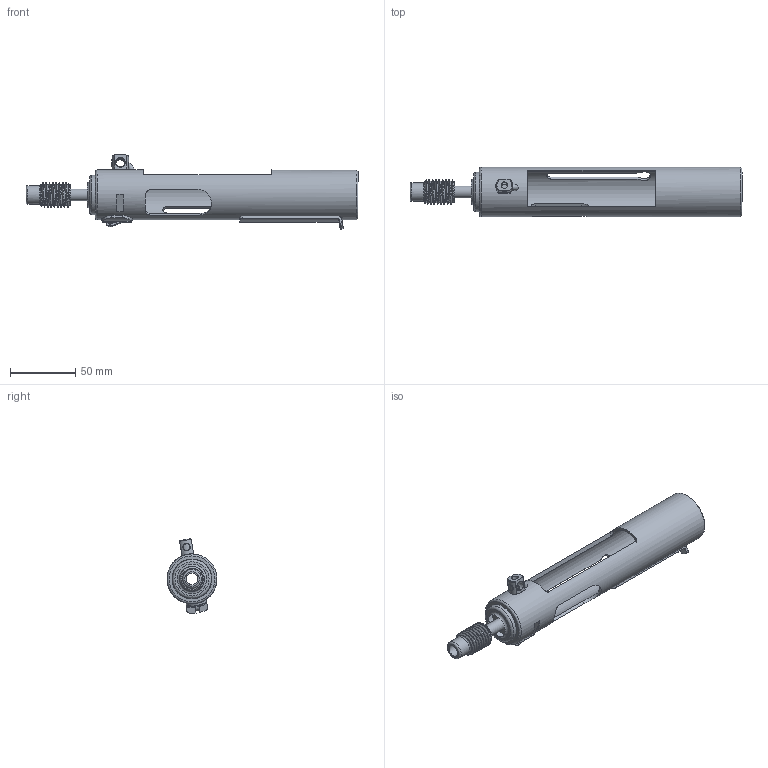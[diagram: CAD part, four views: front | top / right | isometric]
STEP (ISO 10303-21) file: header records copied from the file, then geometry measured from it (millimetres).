
FILE_DESCRIPTION(/* description */ (''),/* implementation_level */ '2;1');
FILE_NAME(/* name */ 'TwoStripedMini.step',/* time_stamp */ '2025-06-07T20:25:17-04:00',/* author */ (''),/* organization */ (''),/* preprocessor_version */ 'ST-DEVELOPER v20.1',/* originating_system */ 'Autodesk Translation Framework v14.10.0.0',/* authorisation */ '');
FILE_SCHEMA (('AUTOMOTIVE_DESIGN { 1 0 10303 214 3 1 1 }'));
Length unit declared in the file: millimetre
Products named in the file (1): Mock Up Tec 9
Bounding box: 253.7 x 38.08 x 57.02 mm (x, y, z)
Volume: 54432.3 mm3; surface area: 48444.3 mm2
Topology: 5 solids, 5 shells, 130 faces, 344 edges, 230 vertices
Faces by surface type: cylinder 57, plane 45, bspline 13, cone 9, torus 6
Full cylindrical faces by diameter (mm): 5 x2, 5.5 x1, 7 x1, 8 x1, 9 x1, 14.2 x1, 16.025 x8, 18.885 x7, 34.1 x1, 38.1 x1
Entity records: 9928 total; most frequent: CARTESIAN_POINT 6807, ORIENTED_EDGE 688, DIRECTION 551, EDGE_CURVE 344, VERTEX_POINT 230, AXIS2_PLACEMENT_3D 207, EDGE_LOOP 154, LINE 137
